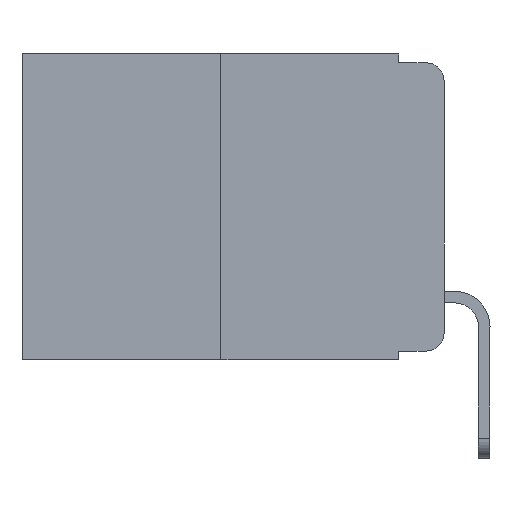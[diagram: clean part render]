
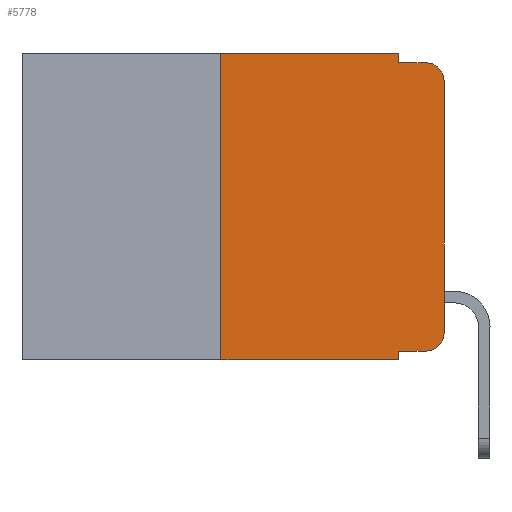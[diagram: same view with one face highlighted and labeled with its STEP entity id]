
A CAD part, left-side view. The second image highlights one B-rep face of the part: STEP entity #5778.
In plain terms, the highlighted planar face has unit normal (-1, 0, 0).
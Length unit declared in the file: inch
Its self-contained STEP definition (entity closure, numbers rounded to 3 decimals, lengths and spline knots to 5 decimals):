
#26 = EDGE_CURVE ( 'NONE', #8114, #7080, #6335, .T. ) ;
#149 = AXIS2_PLACEMENT_3D ( 'NONE', #944, #336, #10261 ) ;
#259 = EDGE_CURVE ( 'NONE', #1562, #704, #6040, .T. ) ;
#336 = DIRECTION ( 'NONE',  ( 1., 0., 0. ) ) ;
#532 = DIRECTION ( 'NONE',  ( 0., 0., -1. ) ) ;
#561 = LINE ( 'NONE', #3791, #5130 ) ;
#566 = ORIENTED_EDGE ( 'NONE', *, *, #4638, .F. ) ;
#704 = VERTEX_POINT ( 'NONE', #1663 ) ;
#903 = PLANE ( 'NONE',  #149 ) ;
#944 = CARTESIAN_POINT ( 'NONE',  ( 0., 0.473, 0. ) ) ;
#956 = AXIS2_PLACEMENT_3D ( 'NONE', #1517, #7045, #4331 ) ;
#1517 = CARTESIAN_POINT ( 'NONE',  ( 0., 0.02, -0.03 ) ) ;
#1562 = VERTEX_POINT ( 'NONE', #4898 ) ;
#1663 = CARTESIAN_POINT ( 'NONE',  ( 0., 0.02, -0.01 ) ) ;
#1857 = EDGE_CURVE ( 'NONE', #9162, #7080, #10756, .T. ) ;
#2200 = ORIENTED_EDGE ( 'NONE', *, *, #5417, .F. ) ;
#2346 = CARTESIAN_POINT ( 'NONE',  ( 0., 0.051, 0. ) ) ;
#2753 = DIRECTION ( 'NONE',  ( 0., 0., -1. ) ) ;
#2806 = LINE ( 'NONE', #10808, #5660 ) ;
#2904 = LINE ( 'NONE', #11646, #11635 ) ;
#3188 = VERTEX_POINT ( 'NONE', #9334 ) ;
#3791 = CARTESIAN_POINT ( 'NONE',  ( 0., 0.051, -0.333 ) ) ;
#4331 = DIRECTION ( 'NONE',  ( 0., 0., -1. ) ) ;
#4486 = ORIENTED_EDGE ( 'NONE', *, *, #259, .F. ) ;
#4517 = CARTESIAN_POINT ( 'NONE',  ( 0., 0.02, -0.313 ) ) ;
#4547 = ORIENTED_EDGE ( 'NONE', *, *, #6783, .F. ) ;
#4638 = EDGE_CURVE ( 'NONE', #3188, #1562, #10678, .T. ) ;
#4868 = CARTESIAN_POINT ( 'NONE',  ( 0., 0.02, -0.333 ) ) ;
#4898 = CARTESIAN_POINT ( 'NONE',  ( 0., 0.051, -0.01 ) ) ;
#5130 = VECTOR ( 'NONE', #9312, 39.37008 ) ;
#5230 = ORIENTED_EDGE ( 'NONE', *, *, #9429, .T. ) ;
#5259 = VECTOR ( 'NONE', #6721, 39.37008 ) ;
#5261 = CARTESIAN_POINT ( 'NONE',  ( 0., 0.051, -0.01 ) ) ;
#5417 = EDGE_CURVE ( 'NONE', #5420, #3188, #2806, .T. ) ;
#5420 = VERTEX_POINT ( 'NONE', #10960 ) ;
#5475 = EDGE_CURVE ( 'NONE', #11019, #7377, #6194, .T. ) ;
#5596 = CARTESIAN_POINT ( 'NONE',  ( 0., 0.051, -0.343 ) ) ;
#5657 = ORIENTED_EDGE ( 'NONE', *, *, #10068, .T. ) ;
#5660 = VECTOR ( 'NONE', #7218, 39.37008 ) ;
#5778 = ADVANCED_FACE ( 'NONE', ( #7047 ), #903, .F. ) ;
#5946 = CARTESIAN_POINT ( 'NONE',  ( 0., 0.25, -0.343 ) ) ;
#6040 = LINE ( 'NONE', #5261, #9346 ) ;
#6053 = CARTESIAN_POINT ( 'NONE',  ( 0., 0.051, 0. ) ) ;
#6161 = EDGE_LOOP ( 'NONE', ( #5657, #11592, #4486, #566, #2200, #4547, #10737, #6786, #5230, #10329 ) ) ;
#6194 = CIRCLE ( 'NONE', #6869, 0.02 ) ;
#6335 = LINE ( 'NONE', #6053, #7335 ) ;
#6503 = VERTEX_POINT ( 'NONE', #9925 ) ;
#6721 = DIRECTION ( 'NONE',  ( 0., 0., 1. ) ) ;
#6783 = EDGE_CURVE ( 'NONE', #9162, #5420, #2904, .T. ) ;
#6786 = ORIENTED_EDGE ( 'NONE', *, *, #26, .F. ) ;
#6869 = AXIS2_PLACEMENT_3D ( 'NONE', #4517, #8216, #2753 ) ;
#7045 = DIRECTION ( 'NONE',  ( -1., 0., 0. ) ) ;
#7047 = FACE_OUTER_BOUND ( 'NONE', #6161, .T. ) ;
#7080 = VERTEX_POINT ( 'NONE', #5596 ) ;
#7218 = DIRECTION ( 'NONE',  ( 0., -1., 0. ) ) ;
#7335 = VECTOR ( 'NONE', #9715, 39.37008 ) ;
#7345 = VECTOR ( 'NONE', #532, 39.37008 ) ;
#7377 = VERTEX_POINT ( 'NONE', #9768 ) ;
#7398 = DIRECTION ( 'NONE',  ( 0., -1., 0. ) ) ;
#8114 = VERTEX_POINT ( 'NONE', #8125 ) ;
#8125 = CARTESIAN_POINT ( 'NONE',  ( 0., 0.051, -0.333 ) ) ;
#8216 = DIRECTION ( 'NONE',  ( -1., 0., 0. ) ) ;
#8420 = CIRCLE ( 'NONE', #956, 0.02 ) ;
#9162 = VERTEX_POINT ( 'NONE', #5946 ) ;
#9285 = CARTESIAN_POINT ( 'NONE',  ( 0., 0.473, -0.343 ) ) ;
#9312 = DIRECTION ( 'NONE',  ( 0., -1., 0. ) ) ;
#9334 = CARTESIAN_POINT ( 'NONE',  ( 0., 0.051, 0. ) ) ;
#9346 = VECTOR ( 'NONE', #11695, 39.37008 ) ;
#9429 = EDGE_CURVE ( 'NONE', #8114, #11019, #561, .T. ) ;
#9443 = CARTESIAN_POINT ( 'NONE',  ( 0., 0., 0. ) ) ;
#9715 = DIRECTION ( 'NONE',  ( 0., 0., -1. ) ) ;
#9723 = LINE ( 'NONE', #9443, #5259 ) ;
#9768 = CARTESIAN_POINT ( 'NONE',  ( 0., 0., -0.313 ) ) ;
#9791 = DIRECTION ( 'NONE',  ( 0., 0., 1. ) ) ;
#9925 = CARTESIAN_POINT ( 'NONE',  ( 0., 0., -0.03 ) ) ;
#10068 = EDGE_CURVE ( 'NONE', #7377, #6503, #9723, .T. ) ;
#10261 = DIRECTION ( 'NONE',  ( 0., 0., -1. ) ) ;
#10329 = ORIENTED_EDGE ( 'NONE', *, *, #5475, .T. ) ;
#10638 = EDGE_CURVE ( 'NONE', #6503, #704, #8420, .T. ) ;
#10678 = LINE ( 'NONE', #2346, #7345 ) ;
#10737 = ORIENTED_EDGE ( 'NONE', *, *, #1857, .T. ) ;
#10756 = LINE ( 'NONE', #9285, #11479 ) ;
#10808 = CARTESIAN_POINT ( 'NONE',  ( 0., 0.473, 0. ) ) ;
#10960 = CARTESIAN_POINT ( 'NONE',  ( 0., 0.25, 0. ) ) ;
#11019 = VERTEX_POINT ( 'NONE', #4868 ) ;
#11479 = VECTOR ( 'NONE', #7398, 39.37008 ) ;
#11592 = ORIENTED_EDGE ( 'NONE', *, *, #10638, .T. ) ;
#11635 = VECTOR ( 'NONE', #9791, 39.37008 ) ;
#11646 = CARTESIAN_POINT ( 'NONE',  ( 0., 0.25, 0. ) ) ;
#11695 = DIRECTION ( 'NONE',  ( 0., -1., 0. ) ) ;
